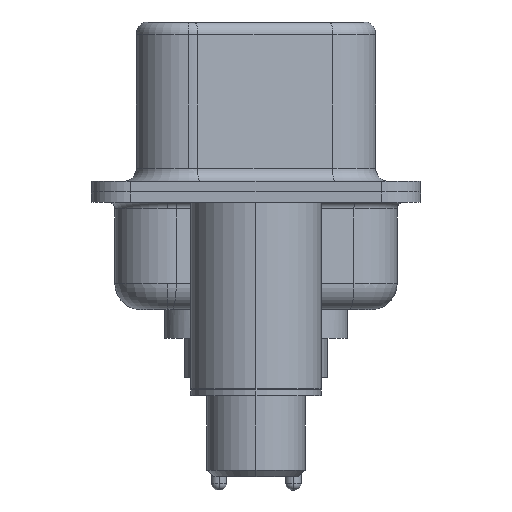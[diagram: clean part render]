
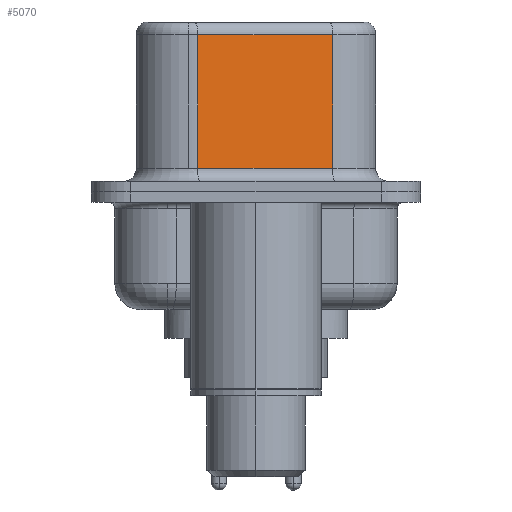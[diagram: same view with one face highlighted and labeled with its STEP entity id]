
A CAD part, left-side view. The second image highlights one B-rep face of the part: STEP entity #5070.
In plain terms, the highlighted planar face has unit normal (-0.985, -0.174, 0).
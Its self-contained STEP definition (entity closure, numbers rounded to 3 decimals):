
#269 = AXIS2_PLACEMENT_3D ( 'NONE', #4707, #1024, #19357 ) ;
#375 = FACE_OUTER_BOUND ( 'NONE', #1724, .T. ) ;
#578 = DIRECTION ( 'NONE',  ( 0.174, -0.985, 0. ) ) ;
#595 = CARTESIAN_POINT ( 'NONE',  ( 4.585, -2.927, 6.52 ) ) ;
#730 = VECTOR ( 'NONE', #16032, 1000. ) ;
#1024 = DIRECTION ( 'NONE',  ( 0.985, 0.174, 0. ) ) ;
#1541 = LINE ( 'NONE', #3244, #730 ) ;
#1724 = EDGE_LOOP ( 'NONE', ( #3014, #12793, #21590, #17016 ) ) ;
#2359 = LINE ( 'NONE', #595, #4946 ) ;
#2591 = VERTEX_POINT ( 'NONE', #5162 ) ;
#3014 = ORIENTED_EDGE ( 'NONE', *, *, #22984, .F. ) ;
#3244 = CARTESIAN_POINT ( 'NONE',  ( 4.585, -2.927, 6.02 ) ) ;
#3666 = EDGE_CURVE ( 'NONE', #20002, #2591, #1541, .T. ) ;
#4364 = EDGE_CURVE ( 'NONE', #2591, #23273, #5299, .T. ) ;
#4597 = EDGE_CURVE ( 'NONE', #23273, #12672, #21580, .T. ) ;
#4707 = CARTESIAN_POINT ( 'NONE',  ( 4.585, -2.927, 6.52 ) ) ;
#4880 = CARTESIAN_POINT ( 'NONE',  ( 3.675, 2.233, 0.9 ) ) ;
#4946 = VECTOR ( 'NONE', #13383, 1000. ) ;
#5070 = ADVANCED_FACE ( 'NONE', ( #375 ), #6473, .F. ) ;
#5162 = CARTESIAN_POINT ( 'NONE',  ( 3.675, 2.233, 6.02 ) ) ;
#5299 = LINE ( 'NONE', #15107, #15883 ) ;
#6473 = PLANE ( 'NONE',  #269 ) ;
#8570 = CARTESIAN_POINT ( 'NONE',  ( 4.585, -2.927, 0.9 ) ) ;
#12672 = VERTEX_POINT ( 'NONE', #8570 ) ;
#12793 = ORIENTED_EDGE ( 'NONE', *, *, #3666, .T. ) ;
#13383 = DIRECTION ( 'NONE',  ( 0., 0., -1. ) ) ;
#14707 = VECTOR ( 'NONE', #578, 1000. ) ;
#14943 = DIRECTION ( 'NONE',  ( 0., 0., -1. ) ) ;
#15107 = CARTESIAN_POINT ( 'NONE',  ( 3.675, 2.233, 6.52 ) ) ;
#15883 = VECTOR ( 'NONE', #14943, 1000. ) ;
#16032 = DIRECTION ( 'NONE',  ( -0.174, 0.985, 0. ) ) ;
#17016 = ORIENTED_EDGE ( 'NONE', *, *, #4597, .T. ) ;
#18111 = CARTESIAN_POINT ( 'NONE',  ( 4.585, -2.927, 6.02 ) ) ;
#19357 = DIRECTION ( 'NONE',  ( -0.174, 0.985, 0. ) ) ;
#20002 = VERTEX_POINT ( 'NONE', #18111 ) ;
#20417 = CARTESIAN_POINT ( 'NONE',  ( 4.585, -2.927, 0.9 ) ) ;
#21580 = LINE ( 'NONE', #20417, #14707 ) ;
#21590 = ORIENTED_EDGE ( 'NONE', *, *, #4364, .T. ) ;
#22984 = EDGE_CURVE ( 'NONE', #20002, #12672, #2359, .T. ) ;
#23273 = VERTEX_POINT ( 'NONE', #4880 ) ;
